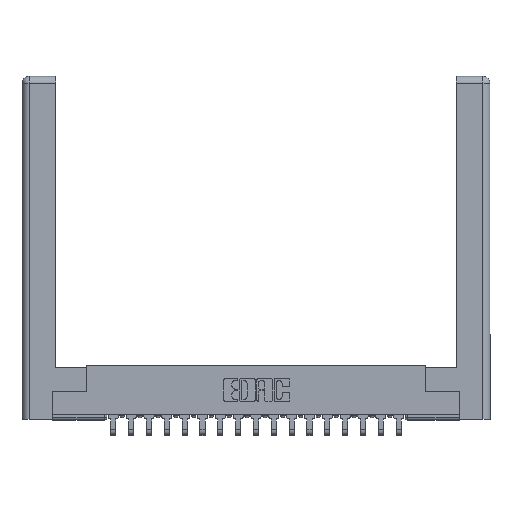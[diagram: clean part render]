
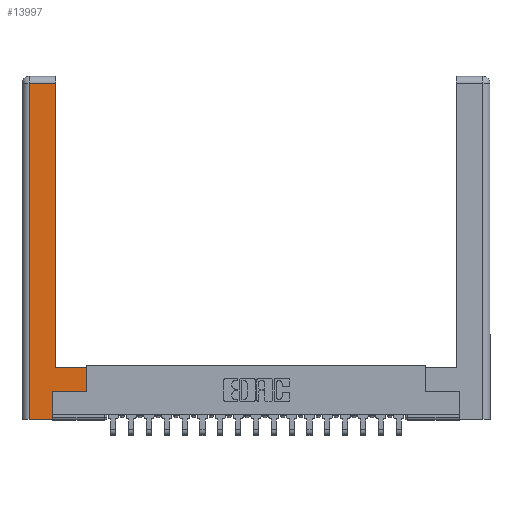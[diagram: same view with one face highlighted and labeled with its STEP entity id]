
A CAD part, top view. The second image highlights one B-rep face of the part: STEP entity #13997.
In plain terms, the highlighted planar face has unit normal (0, 0, 1).
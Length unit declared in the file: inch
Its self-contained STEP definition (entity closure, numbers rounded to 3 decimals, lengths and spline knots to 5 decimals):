
#275 = DIRECTION ( 'NONE',  ( -1., 0., 0. ) ) ;
#339 = LINE ( 'NONE', #5308, #13952 ) ;
#427 = VERTEX_POINT ( 'NONE', #14003 ) ;
#481 = LINE ( 'NONE', #1620, #7913 ) ;
#1012 = CARTESIAN_POINT ( 'NONE',  ( 0.265, 0., 0. ) ) ;
#1082 = DIRECTION ( 'NONE',  ( 1., 0., 0. ) ) ;
#1418 = DIRECTION ( 'NONE',  ( 0., 1., 0. ) ) ;
#1498 = CARTESIAN_POINT ( 'NONE',  ( 0.0615, 2.94, 0. ) ) ;
#1505 = VERTEX_POINT ( 'NONE', #5855 ) ;
#1548 = CARTESIAN_POINT ( 'NONE',  ( 0.0615, 2.94, 0. ) ) ;
#1620 = CARTESIAN_POINT ( 'NONE',  ( 0.0615, 0., 0. ) ) ;
#2784 = LINE ( 'NONE', #18930, #6025 ) ;
#2836 = VERTEX_POINT ( 'NONE', #1498 ) ;
#2980 = CARTESIAN_POINT ( 'NONE',  ( 0.565, 0.245, 0. ) ) ;
#3323 = PLANE ( 'NONE',  #17121 ) ;
#4612 = ORIENTED_EDGE ( 'NONE', *, *, #9140, .T. ) ;
#5308 = CARTESIAN_POINT ( 'NONE',  ( 0.265, 0.245, 0. ) ) ;
#5390 = VERTEX_POINT ( 'NONE', #19231 ) ;
#5475 = LINE ( 'NONE', #12604, #18999 ) ;
#5576 = ORIENTED_EDGE ( 'NONE', *, *, #6496, .T. ) ;
#5693 = LINE ( 'NONE', #2980, #19699 ) ;
#5855 = CARTESIAN_POINT ( 'NONE',  ( 0.295, 2.94, 0. ) ) ;
#6025 = VECTOR ( 'NONE', #9598, 39.37008 ) ;
#6410 = CARTESIAN_POINT ( 'NONE',  ( 0.265, 0.245, 0. ) ) ;
#6496 = EDGE_CURVE ( 'NONE', #427, #19849, #2784, .T. ) ;
#6850 = CARTESIAN_POINT ( 'NONE',  ( 0.295, 0.45, 0. ) ) ;
#7061 = EDGE_CURVE ( 'NONE', #5390, #11687, #19262, .T. ) ;
#7358 = LINE ( 'NONE', #1548, #11311 ) ;
#7439 = ORIENTED_EDGE ( 'NONE', *, *, #7061, .T. ) ;
#7459 = ORIENTED_EDGE ( 'NONE', *, *, #18647, .T. ) ;
#7913 = VECTOR ( 'NONE', #11253, 39.37008 ) ;
#7980 = CARTESIAN_POINT ( 'NONE',  ( 0.295, 3., 0. ) ) ;
#9140 = EDGE_CURVE ( 'NONE', #1505, #2836, #7358, .T. ) ;
#9227 = VERTEX_POINT ( 'NONE', #6410 ) ;
#9598 = DIRECTION ( 'NONE',  ( -1., 0., 0. ) ) ;
#9780 = DIRECTION ( 'NONE',  ( 0., 0., -1. ) ) ;
#10294 = DIRECTION ( 'NONE',  ( 0., 1., 0. ) ) ;
#10319 = ORIENTED_EDGE ( 'NONE', *, *, #15874, .T. ) ;
#10498 = EDGE_CURVE ( 'NONE', #11687, #9227, #339, .T. ) ;
#11253 = DIRECTION ( 'NONE',  ( 0., -1., 0. ) ) ;
#11311 = VECTOR ( 'NONE', #14060, 39.37008 ) ;
#11687 = VERTEX_POINT ( 'NONE', #15931 ) ;
#11730 = LINE ( 'NONE', #7980, #18098 ) ;
#12604 = CARTESIAN_POINT ( 'NONE',  ( 0.565, 0.45, 0. ) ) ;
#12684 = DIRECTION ( 'NONE',  ( 0., 1., 0. ) ) ;
#13224 = EDGE_LOOP ( 'NONE', ( #10319, #4612, #7459, #7439, #13636, #15906, #16810, #5576 ) ) ;
#13253 = EDGE_CURVE ( 'NONE', #17316, #427, #5475, .T. ) ;
#13636 = ORIENTED_EDGE ( 'NONE', *, *, #10498, .T. ) ;
#13952 = VECTOR ( 'NONE', #12684, 39.37008 ) ;
#13997 = ADVANCED_FACE ( 'NONE', ( #18623 ), #3323, .F. ) ;
#14003 = CARTESIAN_POINT ( 'NONE',  ( 0.565, 0.45, 0. ) ) ;
#14060 = DIRECTION ( 'NONE',  ( -1., 0., 0. ) ) ;
#14180 = DIRECTION ( 'NONE',  ( 1., 0., 0. ) ) ;
#14372 = CARTESIAN_POINT ( 'NONE',  ( 0., 0., 0. ) ) ;
#15874 = EDGE_CURVE ( 'NONE', #19849, #1505, #11730, .T. ) ;
#15906 = ORIENTED_EDGE ( 'NONE', *, *, #18866, .T. ) ;
#15931 = CARTESIAN_POINT ( 'NONE',  ( 0.265, 0., 0. ) ) ;
#16775 = CARTESIAN_POINT ( 'NONE',  ( 0.565, 0.245, 0. ) ) ;
#16810 = ORIENTED_EDGE ( 'NONE', *, *, #13253, .T. ) ;
#17121 = AXIS2_PLACEMENT_3D ( 'NONE', #14372, #9780, #275 ) ;
#17316 = VERTEX_POINT ( 'NONE', #16775 ) ;
#17558 = VECTOR ( 'NONE', #1082, 39.37008 ) ;
#18098 = VECTOR ( 'NONE', #10294, 39.37008 ) ;
#18623 = FACE_OUTER_BOUND ( 'NONE', #13224, .T. ) ;
#18647 = EDGE_CURVE ( 'NONE', #2836, #5390, #481, .T. ) ;
#18866 = EDGE_CURVE ( 'NONE', #9227, #17316, #5693, .T. ) ;
#18930 = CARTESIAN_POINT ( 'NONE',  ( 0.295, 0.45, 0. ) ) ;
#18999 = VECTOR ( 'NONE', #1418, 39.37008 ) ;
#19231 = CARTESIAN_POINT ( 'NONE',  ( 0.0615, 0., 0. ) ) ;
#19262 = LINE ( 'NONE', #1012, #17558 ) ;
#19699 = VECTOR ( 'NONE', #14180, 39.37008 ) ;
#19849 = VERTEX_POINT ( 'NONE', #6850 ) ;
